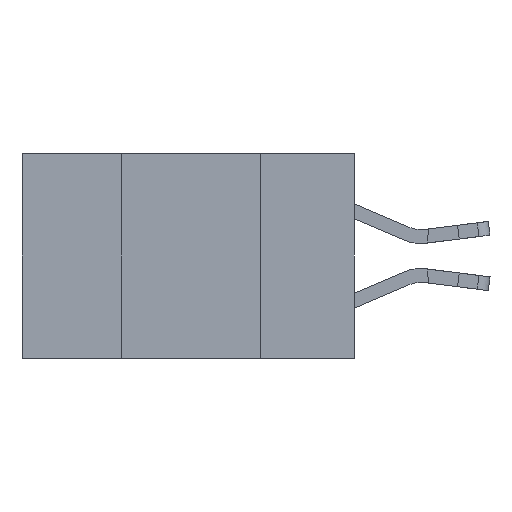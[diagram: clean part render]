
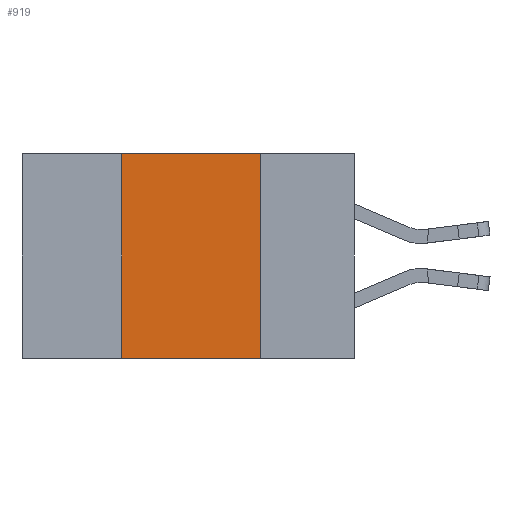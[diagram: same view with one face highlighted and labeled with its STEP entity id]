
A CAD part, left-side view. The second image highlights one B-rep face of the part: STEP entity #919.
In plain terms, the highlighted planar face has unit normal (-1, 0, 0).
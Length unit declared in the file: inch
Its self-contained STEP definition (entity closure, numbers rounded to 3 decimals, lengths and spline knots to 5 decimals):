
#3 = ORIENTED_EDGE ( 'NONE', *, *, #6372, .T. ) ;
#269 = EDGE_CURVE ( 'NONE', #1229, #6187, #4080, .T. ) ;
#919 = ADVANCED_FACE ( 'NONE', ( #4510 ), #11483, .F. ) ;
#1229 = VERTEX_POINT ( 'NONE', #1460 ) ;
#1460 = CARTESIAN_POINT ( 'NONE',  ( 0., 0.17, 0. ) ) ;
#1534 = VECTOR ( 'NONE', #3570, 39.37008 ) ;
#2232 = ORIENTED_EDGE ( 'NONE', *, *, #9714, .F. ) ;
#2809 = CARTESIAN_POINT ( 'NONE',  ( 0., 0.6, 0. ) ) ;
#2907 = CARTESIAN_POINT ( 'NONE',  ( 0., 0.17, -0.37 ) ) ;
#3256 = LINE ( 'NONE', #9803, #5756 ) ;
#3570 = DIRECTION ( 'NONE',  ( 0., 0., -1. ) ) ;
#3628 = CARTESIAN_POINT ( 'NONE',  ( 0., 0.6, 0. ) ) ;
#3644 = DIRECTION ( 'NONE',  ( 0., -1., 0. ) ) ;
#3892 = DIRECTION ( 'NONE',  ( 0., 0., -1. ) ) ;
#4080 = LINE ( 'NONE', #2907, #1534 ) ;
#4130 = EDGE_CURVE ( 'NONE', #5327, #1229, #10998, .T. ) ;
#4510 = FACE_OUTER_BOUND ( 'NONE', #4830, .T. ) ;
#4830 = EDGE_LOOP ( 'NONE', ( #9135, #11538, #2232, #3 ) ) ;
#5327 = VERTEX_POINT ( 'NONE', #7894 ) ;
#5459 = CARTESIAN_POINT ( 'NONE',  ( 0., 0.42, -0.37 ) ) ;
#5756 = VECTOR ( 'NONE', #9802, 39.37008 ) ;
#6011 = VECTOR ( 'NONE', #11889, 39.37008 ) ;
#6187 = VERTEX_POINT ( 'NONE', #10064 ) ;
#6372 = EDGE_CURVE ( 'NONE', #6889, #6187, #3256, .T. ) ;
#6376 = VECTOR ( 'NONE', #3644, 39.37008 ) ;
#6889 = VERTEX_POINT ( 'NONE', #8938 ) ;
#7894 = CARTESIAN_POINT ( 'NONE',  ( 0., 0.42, 0. ) ) ;
#8501 = LINE ( 'NONE', #5459, #6011 ) ;
#8938 = CARTESIAN_POINT ( 'NONE',  ( 0., 0.42, -0.37 ) ) ;
#9135 = ORIENTED_EDGE ( 'NONE', *, *, #269, .F. ) ;
#9604 = DIRECTION ( 'NONE',  ( 1., 0., 0. ) ) ;
#9714 = EDGE_CURVE ( 'NONE', #6889, #5327, #8501, .T. ) ;
#9802 = DIRECTION ( 'NONE',  ( 0., -1., 0. ) ) ;
#9803 = CARTESIAN_POINT ( 'NONE',  ( 0., 0.6, -0.37 ) ) ;
#10064 = CARTESIAN_POINT ( 'NONE',  ( 0., 0.17, -0.37 ) ) ;
#10998 = LINE ( 'NONE', #3628, #6376 ) ;
#11222 = AXIS2_PLACEMENT_3D ( 'NONE', #2809, #9604, #3892 ) ;
#11483 = PLANE ( 'NONE',  #11222 ) ;
#11538 = ORIENTED_EDGE ( 'NONE', *, *, #4130, .F. ) ;
#11889 = DIRECTION ( 'NONE',  ( 0., 0., 1. ) ) ;
